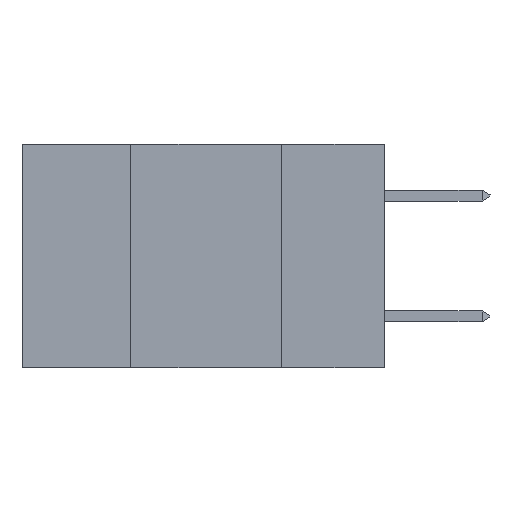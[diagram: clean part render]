
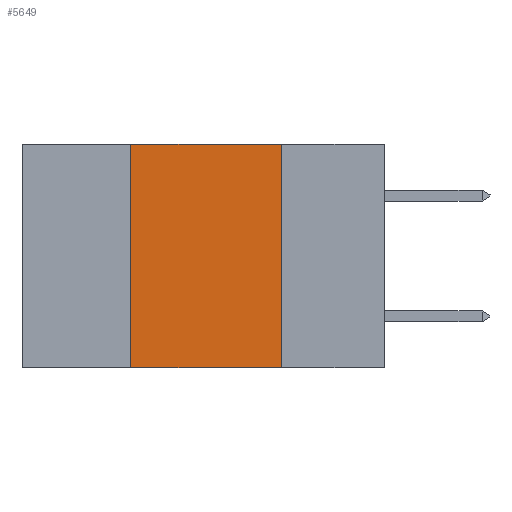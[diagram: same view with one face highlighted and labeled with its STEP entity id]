
A CAD part, left-side view. The second image highlights one B-rep face of the part: STEP entity #5649.
In plain terms, the highlighted planar face has unit normal (-1, 0, 0).
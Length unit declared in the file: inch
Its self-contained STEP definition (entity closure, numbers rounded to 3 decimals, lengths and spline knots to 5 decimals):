
#2613 = PLANE ( 'NONE',  #17925 ) ;
#2765 = ORIENTED_EDGE ( 'NONE', *, *, #9899, .F. ) ;
#3937 = LINE ( 'NONE', #24082, #15102 ) ;
#4231 = DIRECTION ( 'NONE',  ( 0., 0., 1. ) ) ;
#4556 = VECTOR ( 'NONE', #24693, 39.37008 ) ;
#5246 = LINE ( 'NONE', #9150, #4556 ) ;
#5649 = ADVANCED_FACE ( 'NONE', ( #6319 ), #2613, .F. ) ;
#6319 = FACE_OUTER_BOUND ( 'NONE', #11296, .T. ) ;
#7119 = DIRECTION ( 'NONE',  ( 0., 0., -1. ) ) ;
#7780 = VECTOR ( 'NONE', #28596, 39.37008 ) ;
#7927 = CARTESIAN_POINT ( 'NONE',  ( 0., 0.42, 0. ) ) ;
#8537 = DIRECTION ( 'NONE',  ( 0., 0., -1. ) ) ;
#9150 = CARTESIAN_POINT ( 'NONE',  ( 0., 0.6, -0.37 ) ) ;
#9899 = EDGE_CURVE ( 'NONE', #14827, #20572, #16156, .T. ) ;
#10081 = ORIENTED_EDGE ( 'NONE', *, *, #20901, .T. ) ;
#10433 = ORIENTED_EDGE ( 'NONE', *, *, #11801, .F. ) ;
#11217 = CARTESIAN_POINT ( 'NONE',  ( 0., 0.42, -0.37 ) ) ;
#11296 = EDGE_LOOP ( 'NONE', ( #23279, #10433, #2765, #10081 ) ) ;
#11758 = EDGE_CURVE ( 'NONE', #24376, #20863, #3937, .T. ) ;
#11801 = EDGE_CURVE ( 'NONE', #20572, #24376, #13692, .T. ) ;
#13193 = CARTESIAN_POINT ( 'NONE',  ( 0., 0.6, 0. ) ) ;
#13692 = LINE ( 'NONE', #13193, #7780 ) ;
#14827 = VERTEX_POINT ( 'NONE', #11217 ) ;
#15102 = VECTOR ( 'NONE', #8537, 39.37008 ) ;
#16156 = LINE ( 'NONE', #17719, #27144 ) ;
#17719 = CARTESIAN_POINT ( 'NONE',  ( 0., 0.42, 0. ) ) ;
#17925 = AXIS2_PLACEMENT_3D ( 'NONE', #18248, #20458, #7119 ) ;
#18248 = CARTESIAN_POINT ( 'NONE',  ( 0., 0.6, 0. ) ) ;
#20191 = CARTESIAN_POINT ( 'NONE',  ( 0., 0.17, -0.37 ) ) ;
#20458 = DIRECTION ( 'NONE',  ( 1., 0., 0. ) ) ;
#20572 = VERTEX_POINT ( 'NONE', #7927 ) ;
#20863 = VERTEX_POINT ( 'NONE', #20191 ) ;
#20901 = EDGE_CURVE ( 'NONE', #14827, #20863, #5246, .T. ) ;
#23279 = ORIENTED_EDGE ( 'NONE', *, *, #11758, .F. ) ;
#23736 = CARTESIAN_POINT ( 'NONE',  ( 0., 0.17, 0. ) ) ;
#24082 = CARTESIAN_POINT ( 'NONE',  ( 0., 0.17, 0. ) ) ;
#24376 = VERTEX_POINT ( 'NONE', #23736 ) ;
#24693 = DIRECTION ( 'NONE',  ( 0., -1., 0. ) ) ;
#27144 = VECTOR ( 'NONE', #4231, 39.37008 ) ;
#28596 = DIRECTION ( 'NONE',  ( 0., -1., 0. ) ) ;
